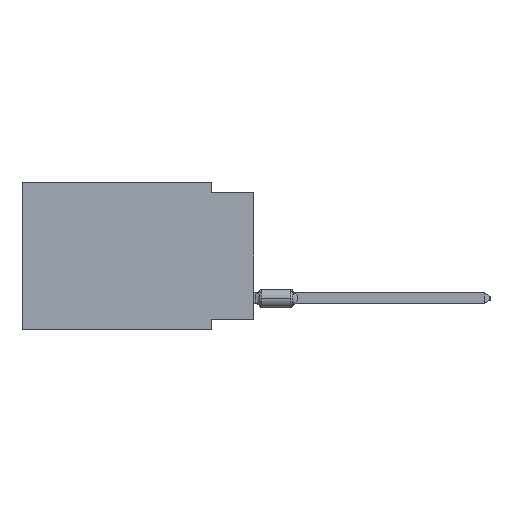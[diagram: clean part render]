
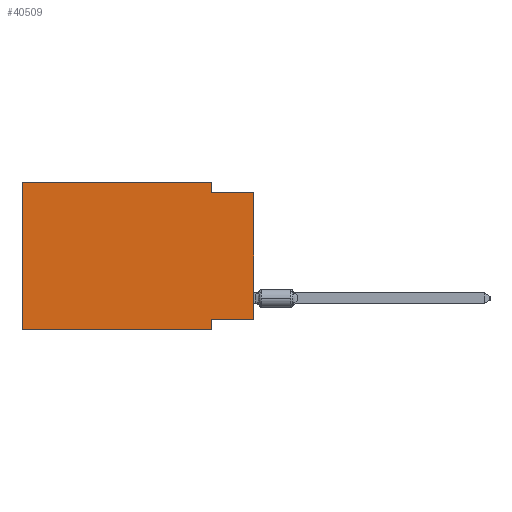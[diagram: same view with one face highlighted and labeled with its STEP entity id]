
A CAD part, left-side view. The second image highlights one B-rep face of the part: STEP entity #40509.
In plain terms, the highlighted planar face has unit normal (-1, 0, 0).
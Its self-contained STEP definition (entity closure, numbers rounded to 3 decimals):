
#800 = CARTESIAN_POINT ( 'NONE',  ( 0., 2.54, 0. ) ) ;
#828 = CARTESIAN_POINT ( 'NONE',  ( 0., 2.54, -8.89 ) ) ;
#1695 = CARTESIAN_POINT ( 'NONE',  ( 0., 2.54, -8.89 ) ) ;
#3811 = CARTESIAN_POINT ( 'NONE',  ( 0., 13.97, 0. ) ) ;
#4235 = DIRECTION ( 'NONE',  ( 0., 0., -1. ) ) ;
#5845 = DIRECTION ( 'NONE',  ( 0., -1., 0. ) ) ;
#6344 = VERTEX_POINT ( 'NONE', #9184 ) ;
#9184 = CARTESIAN_POINT ( 'NONE',  ( 0., 0., -0.635 ) ) ;
#11232 = ORIENTED_EDGE ( 'NONE', *, *, #28385, .T. ) ;
#12909 = DIRECTION ( 'NONE',  ( 0., 0., 1. ) ) ;
#13715 = LINE ( 'NONE', #48918, #24548 ) ;
#18283 = VECTOR ( 'NONE', #12909, 1000. ) ;
#18498 = DIRECTION ( 'NONE',  ( 0., 0., -1. ) ) ;
#19647 = EDGE_CURVE ( 'NONE', #25449, #6344, #13715, .T. ) ;
#21494 = DIRECTION ( 'NONE',  ( 0., -1., 0. ) ) ;
#23120 = FACE_OUTER_BOUND ( 'NONE', #88034, .T. ) ;
#23326 = LINE ( 'NONE', #44352, #72792 ) ;
#24010 = PLANE ( 'NONE',  #71014 ) ;
#24245 = EDGE_CURVE ( 'NONE', #63288, #85325, #81356, .T. ) ;
#24548 = VECTOR ( 'NONE', #21494, 1000. ) ;
#25060 = LINE ( 'NONE', #32361, #89955 ) ;
#25449 = VERTEX_POINT ( 'NONE', #87898 ) ;
#26402 = ORIENTED_EDGE ( 'NONE', *, *, #42588, .F. ) ;
#28385 = EDGE_CURVE ( 'NONE', #40232, #6344, #25060, .T. ) ;
#28667 = VECTOR ( 'NONE', #82407, 1000. ) ;
#30779 = LINE ( 'NONE', #51823, #89622 ) ;
#32361 = CARTESIAN_POINT ( 'NONE',  ( 0., 0., 0. ) ) ;
#32880 = VERTEX_POINT ( 'NONE', #800 ) ;
#33009 = EDGE_CURVE ( 'NONE', #79632, #85325, #63972, .T. ) ;
#38462 = CARTESIAN_POINT ( 'NONE',  ( 0., 2.54, -8.255 ) ) ;
#39093 = ORIENTED_EDGE ( 'NONE', *, *, #24245, .T. ) ;
#40232 = VERTEX_POINT ( 'NONE', #71184 ) ;
#40509 = ADVANCED_FACE ( 'NONE', ( #23120 ), #24010, .F. ) ;
#40799 = LINE ( 'NONE', #89300, #18283 ) ;
#42588 = EDGE_CURVE ( 'NONE', #40232, #79632, #61828, .T. ) ;
#42921 = EDGE_CURVE ( 'NONE', #79120, #32880, #23326, .T. ) ;
#44352 = CARTESIAN_POINT ( 'NONE',  ( 0., 13.97, 0. ) ) ;
#47012 = CARTESIAN_POINT ( 'NONE',  ( 0., 13.97, -8.89 ) ) ;
#48661 = ORIENTED_EDGE ( 'NONE', *, *, #66654, .F. ) ;
#48731 = CARTESIAN_POINT ( 'NONE',  ( 0., 13.97, -8.89 ) ) ;
#48918 = CARTESIAN_POINT ( 'NONE',  ( 0., 0., -0.635 ) ) ;
#51018 = CARTESIAN_POINT ( 'NONE',  ( 0., 13.97, 0. ) ) ;
#51669 = DIRECTION ( 'NONE',  ( 0., -1., 0. ) ) ;
#51823 = CARTESIAN_POINT ( 'NONE',  ( 0., 2.54, 0. ) ) ;
#52728 = VECTOR ( 'NONE', #84554, 1000. ) ;
#56887 = ORIENTED_EDGE ( 'NONE', *, *, #42921, .F. ) ;
#61828 = LINE ( 'NONE', #88837, #28667 ) ;
#63288 = VERTEX_POINT ( 'NONE', #48731 ) ;
#63972 = LINE ( 'NONE', #1695, #52728 ) ;
#66654 = EDGE_CURVE ( 'NONE', #63288, #79120, #40799, .T. ) ;
#68069 = DIRECTION ( 'NONE',  ( 0., 0., 1. ) ) ;
#71014 = AXIS2_PLACEMENT_3D ( 'NONE', #51018, #78933, #18498 ) ;
#71184 = CARTESIAN_POINT ( 'NONE',  ( 0., 0., -8.255 ) ) ;
#72513 = ORIENTED_EDGE ( 'NONE', *, *, #33009, .F. ) ;
#72792 = VECTOR ( 'NONE', #51669, 1000. ) ;
#74785 = VECTOR ( 'NONE', #5845, 1000. ) ;
#77471 = ORIENTED_EDGE ( 'NONE', *, *, #19647, .F. ) ;
#78933 = DIRECTION ( 'NONE',  ( 1., 0., 0. ) ) ;
#79120 = VERTEX_POINT ( 'NONE', #3811 ) ;
#79632 = VERTEX_POINT ( 'NONE', #38462 ) ;
#81056 = ORIENTED_EDGE ( 'NONE', *, *, #81506, .F. ) ;
#81356 = LINE ( 'NONE', #47012, #74785 ) ;
#81506 = EDGE_CURVE ( 'NONE', #32880, #25449, #30779, .T. ) ;
#82407 = DIRECTION ( 'NONE',  ( 0., 1., 0. ) ) ;
#84554 = DIRECTION ( 'NONE',  ( 0., 0., -1. ) ) ;
#85325 = VERTEX_POINT ( 'NONE', #828 ) ;
#87898 = CARTESIAN_POINT ( 'NONE',  ( 0., 2.54, -0.635 ) ) ;
#88034 = EDGE_LOOP ( 'NONE', ( #11232, #77471, #81056, #56887, #48661, #39093, #72513, #26402 ) ) ;
#88837 = CARTESIAN_POINT ( 'NONE',  ( 0., 0., -8.255 ) ) ;
#89300 = CARTESIAN_POINT ( 'NONE',  ( 0., 13.97, 0. ) ) ;
#89622 = VECTOR ( 'NONE', #4235, 1000. ) ;
#89955 = VECTOR ( 'NONE', #68069, 1000. ) ;
